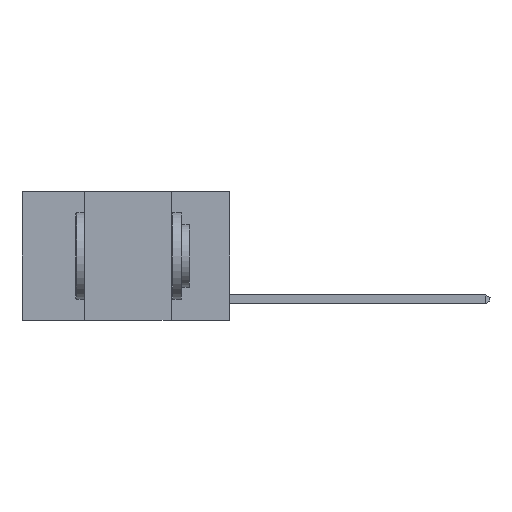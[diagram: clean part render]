
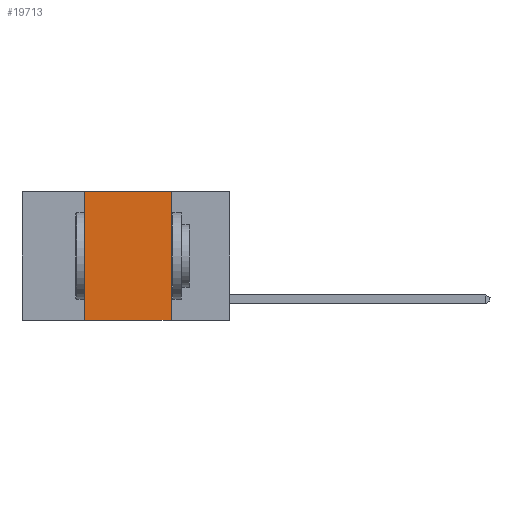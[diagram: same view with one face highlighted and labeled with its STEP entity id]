
A CAD part, left-side view. The second image highlights one B-rep face of the part: STEP entity #19713.
In plain terms, the highlighted planar face has unit normal (-1, 0, 0).
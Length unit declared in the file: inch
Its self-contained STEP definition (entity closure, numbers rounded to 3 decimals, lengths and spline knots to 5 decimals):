
#729 = CARTESIAN_POINT ( 'NONE',  ( 0., 0.6, 0. ) ) ;
#1426 = EDGE_CURVE ( 'NONE', #1653, #8926, #16853, .T. ) ;
#1653 = VERTEX_POINT ( 'NONE', #3787 ) ;
#2057 = AXIS2_PLACEMENT_3D ( 'NONE', #729, #26376, #14596 ) ;
#3787 = CARTESIAN_POINT ( 'NONE',  ( 0., 0.42, 0. ) ) ;
#3823 = ORIENTED_EDGE ( 'NONE', *, *, #27150, .T. ) ;
#3994 = LINE ( 'NONE', #30069, #14546 ) ;
#4614 = ORIENTED_EDGE ( 'NONE', *, *, #23396, .F. ) ;
#6736 = VECTOR ( 'NONE', #30640, 39.37008 ) ;
#6751 = VERTEX_POINT ( 'NONE', #29572 ) ;
#6896 = CARTESIAN_POINT ( 'NONE',  ( 0., 0.42, 0. ) ) ;
#7754 = PLANE ( 'NONE',  #2057 ) ;
#7839 = CARTESIAN_POINT ( 'NONE',  ( 0., 0.6, 0. ) ) ;
#8504 = ORIENTED_EDGE ( 'NONE', *, *, #1426, .F. ) ;
#8926 = VERTEX_POINT ( 'NONE', #28899 ) ;
#9247 = CARTESIAN_POINT ( 'NONE',  ( 0., 0.6, -0.37 ) ) ;
#9943 = VECTOR ( 'NONE', #14523, 39.37008 ) ;
#14523 = DIRECTION ( 'NONE',  ( 0., -1., 0. ) ) ;
#14546 = VECTOR ( 'NONE', #15965, 39.37008 ) ;
#14596 = DIRECTION ( 'NONE',  ( 0., 0., -1. ) ) ;
#15965 = DIRECTION ( 'NONE',  ( 0., 0., -1. ) ) ;
#16725 = LINE ( 'NONE', #9247, #16895 ) ;
#16853 = LINE ( 'NONE', #7839, #9943 ) ;
#16895 = VECTOR ( 'NONE', #26183, 39.37008 ) ;
#16916 = FACE_OUTER_BOUND ( 'NONE', #24299, .T. ) ;
#18241 = ORIENTED_EDGE ( 'NONE', *, *, #30309, .F. ) ;
#19713 = ADVANCED_FACE ( 'NONE', ( #16916 ), #7754, .F. ) ;
#21200 = LINE ( 'NONE', #6896, #6736 ) ;
#22659 = VERTEX_POINT ( 'NONE', #29302 ) ;
#23396 = EDGE_CURVE ( 'NONE', #6751, #1653, #21200, .T. ) ;
#24299 = EDGE_LOOP ( 'NONE', ( #18241, #8504, #4614, #3823 ) ) ;
#26183 = DIRECTION ( 'NONE',  ( 0., -1., 0. ) ) ;
#26376 = DIRECTION ( 'NONE',  ( 1., 0., 0. ) ) ;
#27150 = EDGE_CURVE ( 'NONE', #6751, #22659, #16725, .T. ) ;
#28899 = CARTESIAN_POINT ( 'NONE',  ( 0., 0.17, 0. ) ) ;
#29302 = CARTESIAN_POINT ( 'NONE',  ( 0., 0.17, -0.37 ) ) ;
#29572 = CARTESIAN_POINT ( 'NONE',  ( 0., 0.42, -0.37 ) ) ;
#30069 = CARTESIAN_POINT ( 'NONE',  ( 0., 0.17, 0. ) ) ;
#30309 = EDGE_CURVE ( 'NONE', #8926, #22659, #3994, .T. ) ;
#30640 = DIRECTION ( 'NONE',  ( 0., 0., 1. ) ) ;
